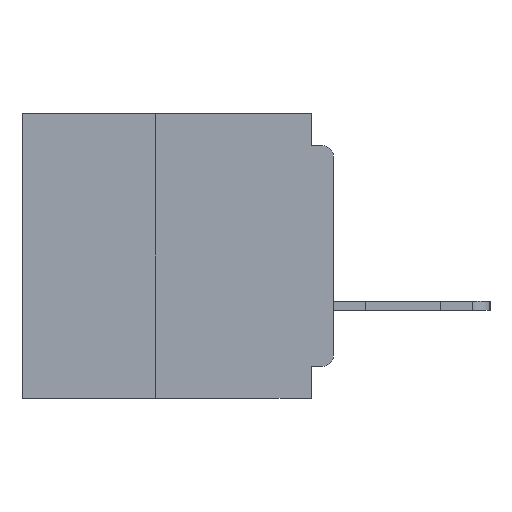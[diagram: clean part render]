
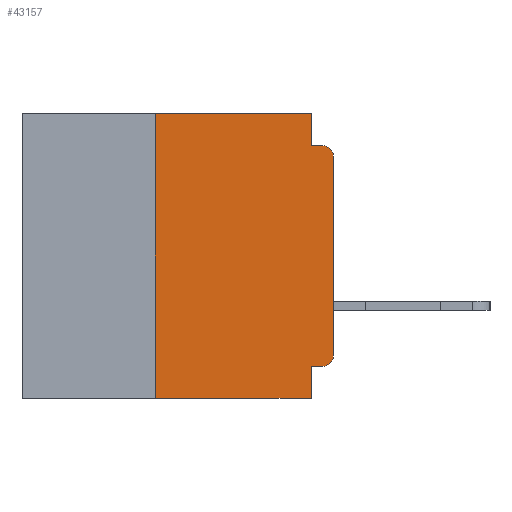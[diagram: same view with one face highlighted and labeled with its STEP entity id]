
A CAD part, left-side view. The second image highlights one B-rep face of the part: STEP entity #43157.
In plain terms, the highlighted planar face has unit normal (-1, 0, 0).
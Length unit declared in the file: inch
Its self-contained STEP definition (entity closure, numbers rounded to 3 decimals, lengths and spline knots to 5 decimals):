
#1183 = DIRECTION ( 'NONE',  ( 0., -1., 0. ) ) ;
#2718 = CARTESIAN_POINT ( 'NONE',  ( 0., 0.25, 0. ) ) ;
#3786 = VERTEX_POINT ( 'NONE', #41222 ) ;
#5235 = CARTESIAN_POINT ( 'NONE',  ( 0., 0.031, -0.4 ) ) ;
#5496 = VECTOR ( 'NONE', #31068, 39.37008 ) ;
#5575 = EDGE_CURVE ( 'NONE', #19201, #43945, #33627, .T. ) ;
#6348 = AXIS2_PLACEMENT_3D ( 'NONE', #7984, #34855, #11833 ) ;
#6424 = CARTESIAN_POINT ( 'NONE',  ( 0., 0.031, -0.4 ) ) ;
#7124 = DIRECTION ( 'NONE',  ( 1., 0., 0. ) ) ;
#7984 = CARTESIAN_POINT ( 'NONE',  ( 0., 0.015, -0.06 ) ) ;
#8190 = VECTOR ( 'NONE', #13916, 39.37008 ) ;
#8234 = AXIS2_PLACEMENT_3D ( 'NONE', #49115, #7124, #34003 ) ;
#9202 = CARTESIAN_POINT ( 'NONE',  ( 0., 0., 0. ) ) ;
#9313 = VERTEX_POINT ( 'NONE', #28702 ) ;
#9552 = CARTESIAN_POINT ( 'NONE',  ( 0., 0.015, -0.34 ) ) ;
#10409 = CARTESIAN_POINT ( 'NONE',  ( 0., 0.031, 0. ) ) ;
#10573 = ORIENTED_EDGE ( 'NONE', *, *, #35039, .F. ) ;
#10668 = ORIENTED_EDGE ( 'NONE', *, *, #21570, .F. ) ;
#11458 = LINE ( 'NONE', #9202, #20479 ) ;
#11833 = DIRECTION ( 'NONE',  ( 0., 0., -1. ) ) ;
#12030 = EDGE_CURVE ( 'NONE', #12885, #33548, #39413, .T. ) ;
#12155 = ORIENTED_EDGE ( 'NONE', *, *, #23697, .T. ) ;
#12885 = VERTEX_POINT ( 'NONE', #21999 ) ;
#13417 = DIRECTION ( 'NONE',  ( 0., 0., -1. ) ) ;
#13916 = DIRECTION ( 'NONE',  ( 0., -1., 0. ) ) ;
#14807 = DIRECTION ( 'NONE',  ( 0., 0., 1. ) ) ;
#15610 = CARTESIAN_POINT ( 'NONE',  ( 0., 0., -0.045 ) ) ;
#16799 = ORIENTED_EDGE ( 'NONE', *, *, #12030, .F. ) ;
#17631 = CARTESIAN_POINT ( 'NONE',  ( 0., 0.437, -0.4 ) ) ;
#17856 = VECTOR ( 'NONE', #38384, 39.37008 ) ;
#19201 = VERTEX_POINT ( 'NONE', #48857 ) ;
#19238 = CARTESIAN_POINT ( 'NONE',  ( 0., 0., -0.34 ) ) ;
#19995 = VECTOR ( 'NONE', #30113, 39.37008 ) ;
#20479 = VECTOR ( 'NONE', #39877, 39.37008 ) ;
#20841 = VECTOR ( 'NONE', #14807, 39.37008 ) ;
#21563 = ORIENTED_EDGE ( 'NONE', *, *, #33845, .T. ) ;
#21570 = EDGE_CURVE ( 'NONE', #9313, #36750, #30032, .T. ) ;
#21594 = CARTESIAN_POINT ( 'NONE',  ( 0., 0.015, -0.045 ) ) ;
#21999 = CARTESIAN_POINT ( 'NONE',  ( 0., 0.031, -0.045 ) ) ;
#23259 = EDGE_CURVE ( 'NONE', #23777, #27345, #31074, .T. ) ;
#23303 = CARTESIAN_POINT ( 'NONE',  ( 0., 0.031, 0. ) ) ;
#23513 = EDGE_CURVE ( 'NONE', #27345, #41854, #29230, .T. ) ;
#23697 = EDGE_CURVE ( 'NONE', #23777, #36750, #39976, .T. ) ;
#23777 = VERTEX_POINT ( 'NONE', #41218 ) ;
#25867 = LINE ( 'NONE', #23303, #5496 ) ;
#26097 = FACE_OUTER_BOUND ( 'NONE', #39153, .T. ) ;
#26826 = EDGE_CURVE ( 'NONE', #19201, #9313, #39148, .T. ) ;
#27345 = VERTEX_POINT ( 'NONE', #2718 ) ;
#27741 = ORIENTED_EDGE ( 'NONE', *, *, #5575, .T. ) ;
#27779 = EDGE_CURVE ( 'NONE', #43945, #3786, #11458, .T. ) ;
#28702 = CARTESIAN_POINT ( 'NONE',  ( 0., 0.031, -0.355 ) ) ;
#29230 = LINE ( 'NONE', #47096, #48348 ) ;
#30032 = LINE ( 'NONE', #5235, #42636 ) ;
#30109 = PLANE ( 'NONE',  #8234 ) ;
#30113 = DIRECTION ( 'NONE',  ( 0., 1., 0. ) ) ;
#30727 = CARTESIAN_POINT ( 'NONE',  ( 0., 0., -0.355 ) ) ;
#30782 = CIRCLE ( 'NONE', #6348, 0.015 ) ;
#31068 = DIRECTION ( 'NONE',  ( 0., 0., -1. ) ) ;
#31074 = LINE ( 'NONE', #33957, #20841 ) ;
#32093 = DIRECTION ( 'NONE',  ( 0., 0., -1. ) ) ;
#33548 = VERTEX_POINT ( 'NONE', #21594 ) ;
#33594 = ORIENTED_EDGE ( 'NONE', *, *, #23259, .F. ) ;
#33627 = CIRCLE ( 'NONE', #34355, 0.015 ) ;
#33845 = EDGE_CURVE ( 'NONE', #3786, #33548, #30782, .T. ) ;
#33925 = ORIENTED_EDGE ( 'NONE', *, *, #26826, .F. ) ;
#33957 = CARTESIAN_POINT ( 'NONE',  ( 0., 0.25, -0.4 ) ) ;
#34003 = DIRECTION ( 'NONE',  ( 0., 0., -1. ) ) ;
#34355 = AXIS2_PLACEMENT_3D ( 'NONE', #9552, #36410, #13417 ) ;
#34855 = DIRECTION ( 'NONE',  ( -1., 0., 0. ) ) ;
#35039 = EDGE_CURVE ( 'NONE', #41854, #12885, #25867, .T. ) ;
#36410 = DIRECTION ( 'NONE',  ( -1., 0., 0. ) ) ;
#36750 = VERTEX_POINT ( 'NONE', #6424 ) ;
#38384 = DIRECTION ( 'NONE',  ( 0., -1., 0. ) ) ;
#39148 = LINE ( 'NONE', #30727, #19995 ) ;
#39153 = EDGE_LOOP ( 'NONE', ( #39510, #21563, #16799, #10573, #41799, #33594, #12155, #10668, #33925, #27741 ) ) ;
#39413 = LINE ( 'NONE', #15610, #17856 ) ;
#39510 = ORIENTED_EDGE ( 'NONE', *, *, #27779, .T. ) ;
#39877 = DIRECTION ( 'NONE',  ( 0., 0., 1. ) ) ;
#39976 = LINE ( 'NONE', #17631, #8190 ) ;
#41218 = CARTESIAN_POINT ( 'NONE',  ( 0., 0.25, -0.4 ) ) ;
#41222 = CARTESIAN_POINT ( 'NONE',  ( 0., 0., -0.06 ) ) ;
#41799 = ORIENTED_EDGE ( 'NONE', *, *, #23513, .F. ) ;
#41854 = VERTEX_POINT ( 'NONE', #10409 ) ;
#42636 = VECTOR ( 'NONE', #32093, 39.37008 ) ;
#43157 = ADVANCED_FACE ( 'NONE', ( #26097 ), #30109, .F. ) ;
#43945 = VERTEX_POINT ( 'NONE', #19238 ) ;
#47096 = CARTESIAN_POINT ( 'NONE',  ( 0., 0.437, 0. ) ) ;
#48348 = VECTOR ( 'NONE', #1183, 39.37008 ) ;
#48857 = CARTESIAN_POINT ( 'NONE',  ( 0., 0.015, -0.355 ) ) ;
#49115 = CARTESIAN_POINT ( 'NONE',  ( 0., 0.437, 0. ) ) ;
